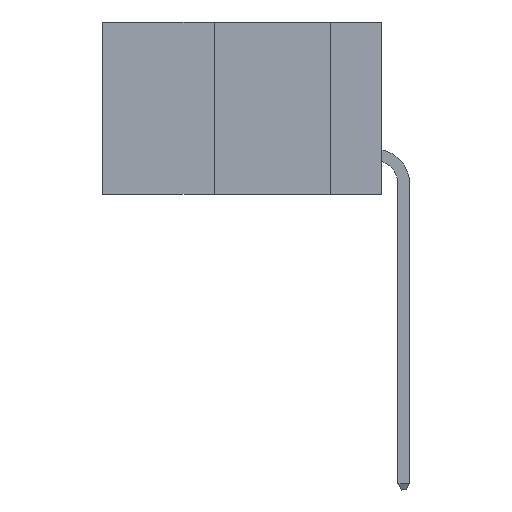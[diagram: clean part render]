
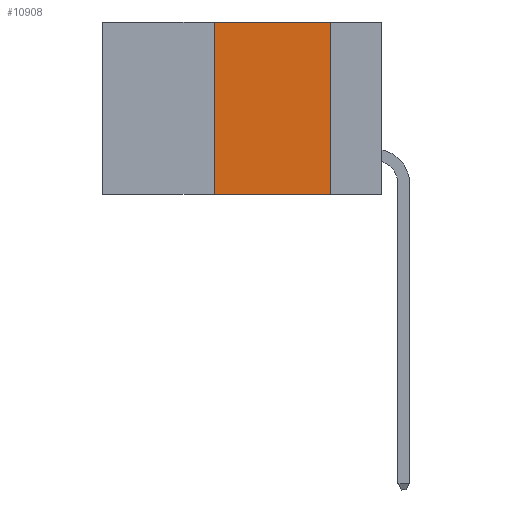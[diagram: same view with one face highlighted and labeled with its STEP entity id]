
A CAD part, left-side view. The second image highlights one B-rep face of the part: STEP entity #10908.
In plain terms, the highlighted planar face has unit normal (-1, 0, 0).
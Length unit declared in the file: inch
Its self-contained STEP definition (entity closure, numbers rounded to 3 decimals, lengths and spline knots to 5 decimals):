
#151 = ORIENTED_EDGE ( 'NONE', *, *, #3375, .F. ) ;
#917 = LINE ( 'NONE', #9854, #13178 ) ;
#1064 = EDGE_CURVE ( 'NONE', #5705, #2612, #1775, .T. ) ;
#1095 = DIRECTION ( 'NONE',  ( 0., 0., -1. ) ) ;
#1603 = CARTESIAN_POINT ( 'NONE',  ( 0., 0.36, -0.37 ) ) ;
#1775 = LINE ( 'NONE', #5727, #14342 ) ;
#1881 = EDGE_CURVE ( 'NONE', #10573, #2180, #2517, .T. ) ;
#2120 = AXIS2_PLACEMENT_3D ( 'NONE', #13291, #8522, #1095 ) ;
#2180 = VERTEX_POINT ( 'NONE', #6392 ) ;
#2435 = CARTESIAN_POINT ( 'NONE',  ( 0., 0.36, 0. ) ) ;
#2517 = LINE ( 'NONE', #12680, #15025 ) ;
#2612 = VERTEX_POINT ( 'NONE', #14906 ) ;
#3375 = EDGE_CURVE ( 'NONE', #10573, #5705, #917, .T. ) ;
#3524 = PLANE ( 'NONE',  #2120 ) ;
#4021 = CARTESIAN_POINT ( 'NONE',  ( 0., 0.11, 0. ) ) ;
#5339 = DIRECTION ( 'NONE',  ( 0., -1., 0. ) ) ;
#5705 = VERTEX_POINT ( 'NONE', #2435 ) ;
#5727 = CARTESIAN_POINT ( 'NONE',  ( 0., 0.6, 0. ) ) ;
#6392 = CARTESIAN_POINT ( 'NONE',  ( 0., 0.11, -0.37 ) ) ;
#7470 = EDGE_LOOP ( 'NONE', ( #14209, #15364, #151, #9686 ) ) ;
#8522 = DIRECTION ( 'NONE',  ( 1., 0., 0. ) ) ;
#9092 = VECTOR ( 'NONE', #14915, 39.37008 ) ;
#9628 = DIRECTION ( 'NONE',  ( 0., 0., 1. ) ) ;
#9686 = ORIENTED_EDGE ( 'NONE', *, *, #1881, .T. ) ;
#9854 = CARTESIAN_POINT ( 'NONE',  ( 0., 0.36, 0. ) ) ;
#10356 = FACE_OUTER_BOUND ( 'NONE', #7470, .T. ) ;
#10573 = VERTEX_POINT ( 'NONE', #1603 ) ;
#10908 = ADVANCED_FACE ( 'NONE', ( #10356 ), #3524, .F. ) ;
#12435 = DIRECTION ( 'NONE',  ( 0., -1., 0. ) ) ;
#12641 = LINE ( 'NONE', #4021, #9092 ) ;
#12680 = CARTESIAN_POINT ( 'NONE',  ( 0., 0.6, -0.37 ) ) ;
#13178 = VECTOR ( 'NONE', #9628, 39.37008 ) ;
#13291 = CARTESIAN_POINT ( 'NONE',  ( 0., 0.6, 0. ) ) ;
#14209 = ORIENTED_EDGE ( 'NONE', *, *, #15277, .F. ) ;
#14342 = VECTOR ( 'NONE', #5339, 39.37008 ) ;
#14906 = CARTESIAN_POINT ( 'NONE',  ( 0., 0.11, 0. ) ) ;
#14915 = DIRECTION ( 'NONE',  ( 0., 0., -1. ) ) ;
#15025 = VECTOR ( 'NONE', #12435, 39.37008 ) ;
#15277 = EDGE_CURVE ( 'NONE', #2612, #2180, #12641, .T. ) ;
#15364 = ORIENTED_EDGE ( 'NONE', *, *, #1064, .F. ) ;
